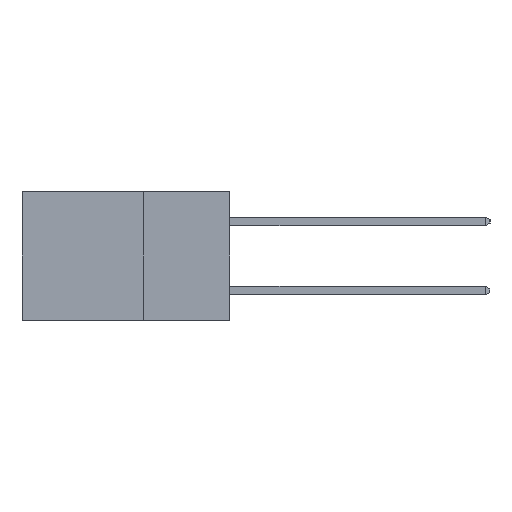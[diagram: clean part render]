
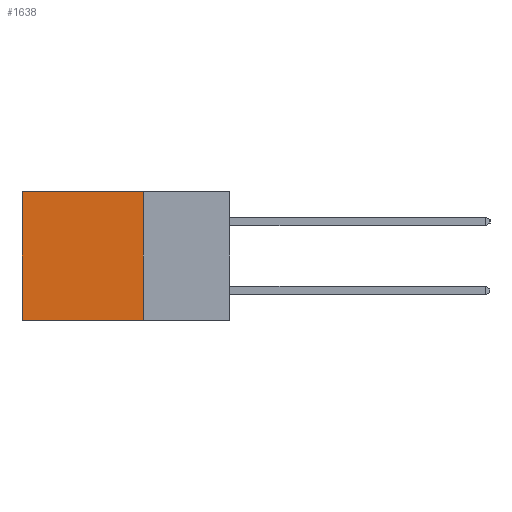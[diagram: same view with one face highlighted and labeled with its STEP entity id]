
A CAD part, left-side view. The second image highlights one B-rep face of the part: STEP entity #1638.
In plain terms, the highlighted planar face has unit normal (-1, 0, 0).
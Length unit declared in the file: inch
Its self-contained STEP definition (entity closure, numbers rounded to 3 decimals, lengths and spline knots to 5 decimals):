
#64 = ORIENTED_EDGE ( 'NONE', *, *, #5374, .T. ) ;
#233 = DIRECTION ( 'NONE',  ( 0., 0., -1. ) ) ;
#296 = LINE ( 'NONE', #12302, #13640 ) ;
#730 = ORIENTED_EDGE ( 'NONE', *, *, #11962, .T. ) ;
#1320 = CARTESIAN_POINT ( 'NONE',  ( 0.298, 0.25, 0. ) ) ;
#1562 = EDGE_LOOP ( 'NONE', ( #730, #1975, #10562, #64 ) ) ;
#1638 = ADVANCED_FACE ( 'NONE', ( #2131 ), #5017, .F. ) ;
#1861 = CARTESIAN_POINT ( 'NONE',  ( 0.298, 0.25, 0. ) ) ;
#1975 = ORIENTED_EDGE ( 'NONE', *, *, #2930, .F. ) ;
#2131 = FACE_OUTER_BOUND ( 'NONE', #1562, .T. ) ;
#2254 = VECTOR ( 'NONE', #6794, 39.37008 ) ;
#2378 = DIRECTION ( 'NONE',  ( 0., 1., 0. ) ) ;
#2529 = CARTESIAN_POINT ( 'NONE',  ( 0.298, 0.25, -0.37 ) ) ;
#2583 = LINE ( 'NONE', #13490, #2254 ) ;
#2930 = EDGE_CURVE ( 'NONE', #11452, #9616, #2583, .T. ) ;
#3001 = DIRECTION ( 'NONE',  ( 0., 0., -1. ) ) ;
#3639 = VERTEX_POINT ( 'NONE', #1861 ) ;
#4125 = EDGE_CURVE ( 'NONE', #3639, #11452, #10259, .T. ) ;
#4829 = CARTESIAN_POINT ( 'NONE',  ( 0.298, 0.25, 0. ) ) ;
#5017 = PLANE ( 'NONE',  #6581 ) ;
#5213 = LINE ( 'NONE', #12908, #12888 ) ;
#5374 = EDGE_CURVE ( 'NONE', #3639, #8133, #296, .T. ) ;
#5404 = VECTOR ( 'NONE', #6073, 39.37008 ) ;
#6073 = DIRECTION ( 'NONE',  ( 0., 0., -1. ) ) ;
#6581 = AXIS2_PLACEMENT_3D ( 'NONE', #4829, #8357, #3001 ) ;
#6794 = DIRECTION ( 'NONE',  ( 0., 1., 0. ) ) ;
#7195 = CARTESIAN_POINT ( 'NONE',  ( 0.298, 0.6, -0.37 ) ) ;
#7949 = CARTESIAN_POINT ( 'NONE',  ( 0.298, 0.6, 0. ) ) ;
#8133 = VERTEX_POINT ( 'NONE', #7949 ) ;
#8357 = DIRECTION ( 'NONE',  ( 1., 0., 0. ) ) ;
#9616 = VERTEX_POINT ( 'NONE', #7195 ) ;
#10259 = LINE ( 'NONE', #1320, #5404 ) ;
#10562 = ORIENTED_EDGE ( 'NONE', *, *, #4125, .F. ) ;
#11452 = VERTEX_POINT ( 'NONE', #2529 ) ;
#11962 = EDGE_CURVE ( 'NONE', #8133, #9616, #5213, .T. ) ;
#12302 = CARTESIAN_POINT ( 'NONE',  ( 0.298, 0.25, 0. ) ) ;
#12888 = VECTOR ( 'NONE', #233, 39.37008 ) ;
#12908 = CARTESIAN_POINT ( 'NONE',  ( 0.298, 0.6, 0. ) ) ;
#13490 = CARTESIAN_POINT ( 'NONE',  ( 0.298, 0.25, -0.37 ) ) ;
#13640 = VECTOR ( 'NONE', #2378, 39.37008 ) ;
